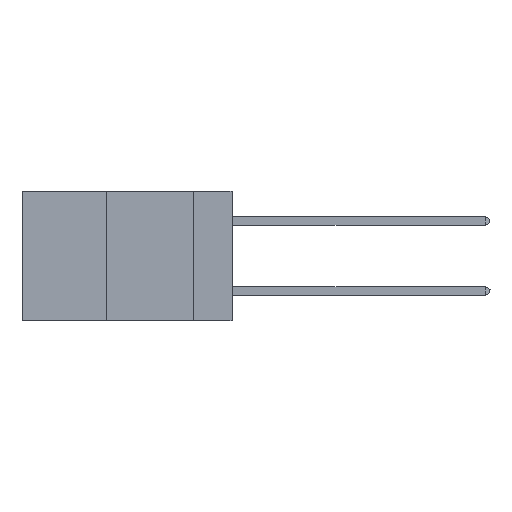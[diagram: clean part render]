
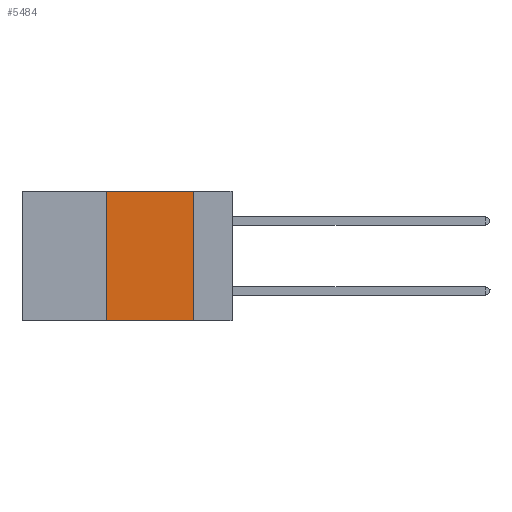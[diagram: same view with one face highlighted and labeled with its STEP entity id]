
A CAD part, left-side view. The second image highlights one B-rep face of the part: STEP entity #5484.
In plain terms, the highlighted planar face has unit normal (-1, 0, 0).
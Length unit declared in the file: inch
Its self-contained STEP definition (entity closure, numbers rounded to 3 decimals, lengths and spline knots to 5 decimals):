
#774 = ORIENTED_EDGE ( 'NONE', *, *, #7926, .F. ) ;
#1132 = VERTEX_POINT ( 'NONE', #13708 ) ;
#1215 = VECTOR ( 'NONE', #2384, 39.37008 ) ;
#1627 = CARTESIAN_POINT ( 'NONE',  ( 0., 0.11, 0. ) ) ;
#2378 = VERTEX_POINT ( 'NONE', #29523 ) ;
#2384 = DIRECTION ( 'NONE',  ( 0., 0., 1. ) ) ;
#4306 = EDGE_CURVE ( 'NONE', #2378, #25174, #17101, .T. ) ;
#4728 = FACE_OUTER_BOUND ( 'NONE', #16493, .T. ) ;
#5228 = EDGE_CURVE ( 'NONE', #20777, #2378, #18604, .T. ) ;
#5484 = ADVANCED_FACE ( 'NONE', ( #4728 ), #18009, .F. ) ;
#7926 = EDGE_CURVE ( 'NONE', #25174, #1132, #16031, .T. ) ;
#10336 = CARTESIAN_POINT ( 'NONE',  ( 0., 0.36, 0. ) ) ;
#10695 = CARTESIAN_POINT ( 'NONE',  ( 0., 0.11, 0. ) ) ;
#11513 = LINE ( 'NONE', #27328, #13451 ) ;
#12096 = ORIENTED_EDGE ( 'NONE', *, *, #4306, .F. ) ;
#13451 = VECTOR ( 'NONE', #13757, 39.37008 ) ;
#13708 = CARTESIAN_POINT ( 'NONE',  ( 0., 0.11, -0.37 ) ) ;
#13757 = DIRECTION ( 'NONE',  ( 0., -1., 0. ) ) ;
#14524 = DIRECTION ( 'NONE',  ( 0., -1., 0. ) ) ;
#14832 = EDGE_CURVE ( 'NONE', #20777, #1132, #11513, .T. ) ;
#16031 = LINE ( 'NONE', #10695, #17736 ) ;
#16493 = EDGE_LOOP ( 'NONE', ( #774, #12096, #18353, #30026 ) ) ;
#17101 = LINE ( 'NONE', #24686, #21583 ) ;
#17736 = VECTOR ( 'NONE', #18452, 39.37008 ) ;
#17786 = CARTESIAN_POINT ( 'NONE',  ( 0., 0.36, -0.37 ) ) ;
#17845 = CARTESIAN_POINT ( 'NONE',  ( 0., 0.6, 0. ) ) ;
#18009 = PLANE ( 'NONE',  #22139 ) ;
#18353 = ORIENTED_EDGE ( 'NONE', *, *, #5228, .F. ) ;
#18452 = DIRECTION ( 'NONE',  ( 0., 0., -1. ) ) ;
#18604 = LINE ( 'NONE', #10336, #1215 ) ;
#20777 = VERTEX_POINT ( 'NONE', #17786 ) ;
#21583 = VECTOR ( 'NONE', #14524, 39.37008 ) ;
#22139 = AXIS2_PLACEMENT_3D ( 'NONE', #17845, #25589, #26260 ) ;
#24686 = CARTESIAN_POINT ( 'NONE',  ( 0., 0.6, 0. ) ) ;
#25174 = VERTEX_POINT ( 'NONE', #1627 ) ;
#25589 = DIRECTION ( 'NONE',  ( 1., 0., 0. ) ) ;
#26260 = DIRECTION ( 'NONE',  ( 0., 0., -1. ) ) ;
#27328 = CARTESIAN_POINT ( 'NONE',  ( 0., 0.6, -0.37 ) ) ;
#29523 = CARTESIAN_POINT ( 'NONE',  ( 0., 0.36, 0. ) ) ;
#30026 = ORIENTED_EDGE ( 'NONE', *, *, #14832, .T. ) ;
